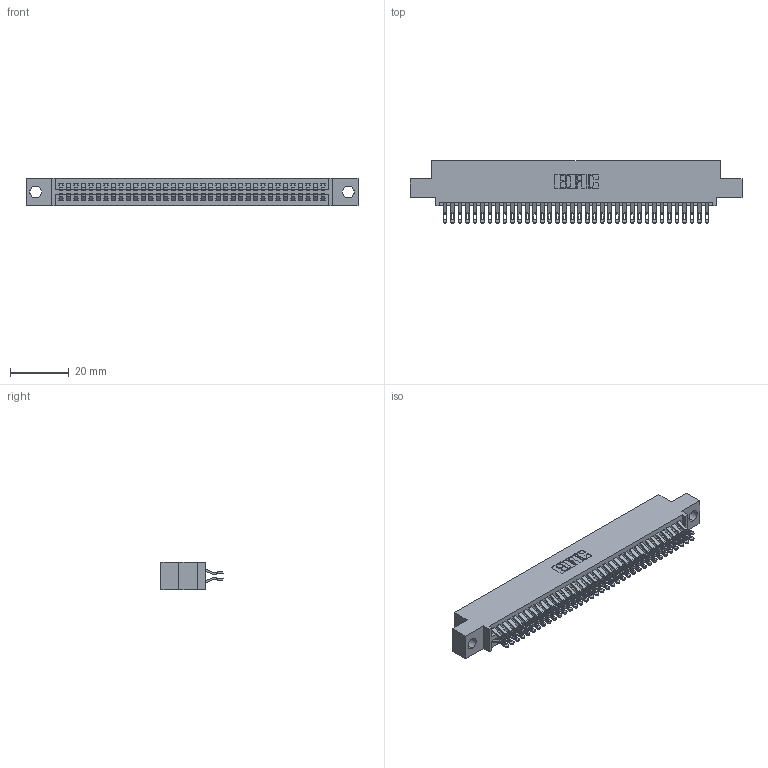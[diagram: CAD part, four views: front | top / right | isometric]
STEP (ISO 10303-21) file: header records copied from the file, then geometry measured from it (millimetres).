
FILE_DESCRIPTION (( 'STEP AP203' ), '1' );
FILE_NAME ('395-072-555-504.STEP', '2018-11-27T15:06:58', ( '' ), ( '' ), 'SwSTEP 2.0', 'SolidWorks 2016', '' );
FILE_SCHEMA (( 'CONFIG_CONTROL_DESIGN' ));
Length unit declared in the file: inch
Products named in the file (3): 345-292-001_555 Tail; 395-072-555-504; 345 Part_0.110 Offset - 0.156 Dia-TH
Assembly tree (73 placements, depth 2):
  395-072-555-504
    345 Part_0.110 Offset - 0.156 Dia-TH
    345-292-001_555 Tail  x72
Bounding box: 112.65 x 21.13 x 9.4 mm (x, y, z)
Volume: 10934.8 mm3; surface area: 16681.6 mm2
Topology: 73 solids, 73 shells, 4162 faces, 13097 edges, 8730 vertices
Faces by surface type: plane 2316, cylinder 1846
Entity records: 29515 total; most frequent: CARTESIAN_POINT 4990, ORIENTED_EDGE 4894, DIRECTION 4375, EDGE_CURVE 2447, VECTOR 2151, LINE 2151, VERTEX_POINT 1630, AXIS2_PLACEMENT_3D 1112
